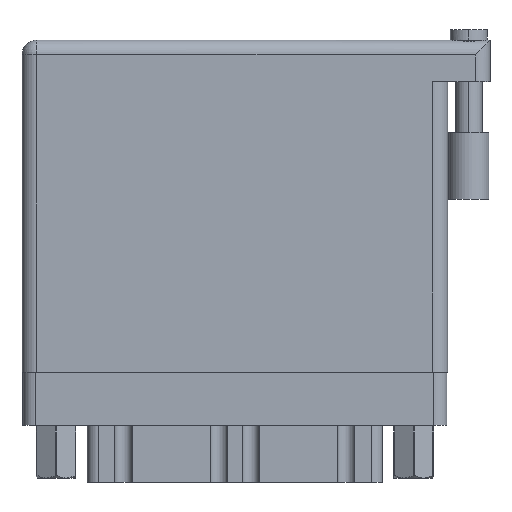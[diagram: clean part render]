
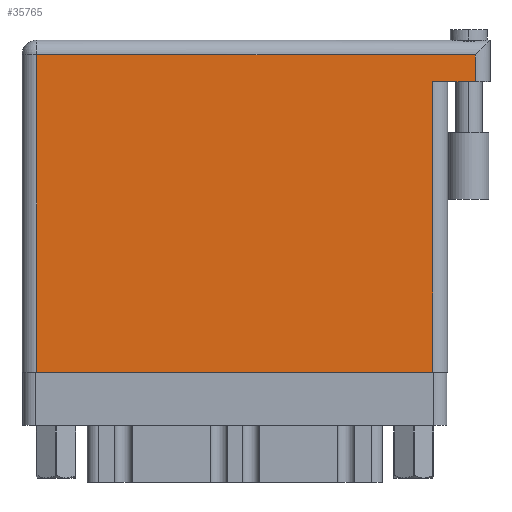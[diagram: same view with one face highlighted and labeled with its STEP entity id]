
A CAD part, front view. The second image highlights one B-rep face of the part: STEP entity #35765.
In plain terms, the highlighted face is planar.
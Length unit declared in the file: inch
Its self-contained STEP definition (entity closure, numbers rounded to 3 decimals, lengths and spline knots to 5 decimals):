
#2361 = EDGE_CURVE ( 'NONE', #39346, #3116, #14489, .T. ) ;
#2556 = CARTESIAN_POINT ( 'NONE',  ( 2.138, 1.496, 0. ) ) ;
#3116 = VERTEX_POINT ( 'NONE', #10343 ) ;
#3982 = ORIENTED_EDGE ( 'NONE', *, *, #2361, .T. ) ;
#4820 = DIRECTION ( 'NONE',  ( -1., 0., 0. ) ) ;
#5134 = ORIENTED_EDGE ( 'NONE', *, *, #29585, .T. ) ;
#6786 = LINE ( 'NONE', #9897, #29963 ) ;
#9897 = CARTESIAN_POINT ( 'NONE',  ( 2.138, 1.566, 0. ) ) ;
#10343 = CARTESIAN_POINT ( 'NONE',  ( 0.07, 0., 0. ) ) ;
#10367 = DIRECTION ( 'NONE',  ( 0., 1., 0. ) ) ;
#11183 = VECTOR ( 'NONE', #23155, 39.37008 ) ;
#11852 = VERTEX_POINT ( 'NONE', #28363 ) ;
#12540 = CARTESIAN_POINT ( 'NONE',  ( 0.07, 0., 0. ) ) ;
#12812 = AXIS2_PLACEMENT_3D ( 'NONE', #23772, #31149, #42120 ) ;
#12913 = CARTESIAN_POINT ( 'NONE',  ( 2.138, 1.369, 0. ) ) ;
#13609 = EDGE_CURVE ( 'NONE', #11852, #25854, #30703, .T. ) ;
#14002 = EDGE_CURVE ( 'NONE', #14150, #35695, #6786, .T. ) ;
#14150 = VERTEX_POINT ( 'NONE', #12913 ) ;
#14489 = LINE ( 'NONE', #12540, #26969 ) ;
#15360 = ORIENTED_EDGE ( 'NONE', *, *, #13609, .T. ) ;
#16921 = LINE ( 'NONE', #20489, #17418 ) ;
#17418 = VECTOR ( 'NONE', #4820, 39.37008 ) ;
#19097 = CARTESIAN_POINT ( 'NONE',  ( 2.208, 1.369, 0. ) ) ;
#20489 = CARTESIAN_POINT ( 'NONE',  ( 0., 1.496, 0. ) ) ;
#23045 = CARTESIAN_POINT ( 'NONE',  ( 0.07, 1.496, 0. ) ) ;
#23155 = DIRECTION ( 'NONE',  ( -1., 0., 0. ) ) ;
#23772 = CARTESIAN_POINT ( 'NONE',  ( 0., 1.566, 0. ) ) ;
#25854 = VERTEX_POINT ( 'NONE', #33189 ) ;
#25899 = ORIENTED_EDGE ( 'NONE', *, *, #41105, .T. ) ;
#26038 = DIRECTION ( 'NONE',  ( 1., 0., 0. ) ) ;
#26969 = VECTOR ( 'NONE', #44957, 39.37008 ) ;
#28363 = CARTESIAN_POINT ( 'NONE',  ( 1.938, 0., 0. ) ) ;
#29585 = EDGE_CURVE ( 'NONE', #35695, #39346, #16921, .T. ) ;
#29963 = VECTOR ( 'NONE', #10367, 39.37008 ) ;
#30703 = LINE ( 'NONE', #45248, #42085 ) ;
#30945 = DIRECTION ( 'NONE',  ( 0., 1., 0. ) ) ;
#31008 = LINE ( 'NONE', #19097, #11183 ) ;
#31149 = DIRECTION ( 'NONE',  ( 0., 0., -1. ) ) ;
#32257 = CARTESIAN_POINT ( 'NONE',  ( 0., 0., 0. ) ) ;
#33189 = CARTESIAN_POINT ( 'NONE',  ( 1.938, 1.369, 0. ) ) ;
#33385 = EDGE_CURVE ( 'NONE', #14150, #25854, #31008, .T. ) ;
#34997 = VECTOR ( 'NONE', #26038, 39.37008 ) ;
#35428 = PLANE ( 'NONE',  #12812 ) ;
#35695 = VERTEX_POINT ( 'NONE', #2556 ) ;
#35765 = ADVANCED_FACE ( 'NONE', ( #41883 ), #35428, .F. ) ;
#35834 = LINE ( 'NONE', #32257, #34997 ) ;
#37971 = ORIENTED_EDGE ( 'NONE', *, *, #14002, .T. ) ;
#39346 = VERTEX_POINT ( 'NONE', #23045 ) ;
#41105 = EDGE_CURVE ( 'NONE', #3116, #11852, #35834, .T. ) ;
#41883 = FACE_OUTER_BOUND ( 'NONE', #43392, .T. ) ;
#42085 = VECTOR ( 'NONE', #30945, 39.37008 ) ;
#42120 = DIRECTION ( 'NONE',  ( -1., 0., 0. ) ) ;
#42383 = ORIENTED_EDGE ( 'NONE', *, *, #33385, .F. ) ;
#43392 = EDGE_LOOP ( 'NONE', ( #25899, #15360, #42383, #37971, #5134, #3982 ) ) ;
#44957 = DIRECTION ( 'NONE',  ( 0., -1., 0. ) ) ;
#45248 = CARTESIAN_POINT ( 'NONE',  ( 1.938, 1.369, 0. ) ) ;
